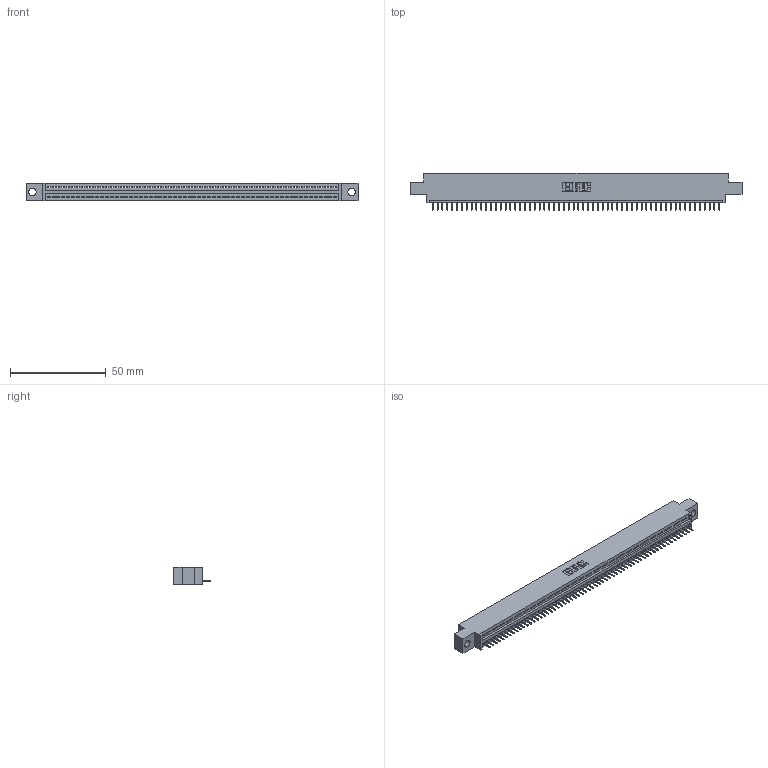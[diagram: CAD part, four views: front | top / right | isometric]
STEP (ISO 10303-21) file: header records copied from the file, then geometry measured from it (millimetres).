
FILE_DESCRIPTION (( 'STEP AP203' ), '1' );
FILE_NAME ('395-060-524-604.STEP', '2019-10-24T11:59:12', ( '' ), ( '' ), 'SwSTEP 2.0', 'SolidWorks 2016', '' );
FILE_SCHEMA (( 'CONFIG_CONTROL_DESIGN' ));
Length unit declared in the file: inch
Products named in the file (3): 395-060-524-604; 345 Part_0.170 Offset - 0.156 Dia-TH; 345-292-001_345-293-124
Assembly tree (61 placements, depth 2):
  395-060-524-604
    345 Part_0.170 Offset - 0.156 Dia-TH
    345-292-001_345-293-124  x60
Bounding box: 173.61 x 19.35 x 9.4 mm (x, y, z)
Volume: 16198.8 mm3; surface area: 20948.8 mm2
Topology: 61 solids, 61 shells, 3850 faces, 11153 edges, 7194 vertices
Faces by surface type: plane 2844, cylinder 1006
Entity records: 42943 total; most frequent: CARTESIAN_POINT 7444, ORIENTED_EDGE 7438, DIRECTION 6475, EDGE_CURVE 3719, VECTOR 3351, LINE 3351, VERTEX_POINT 2474, AXIS2_PLACEMENT_3D 1562
